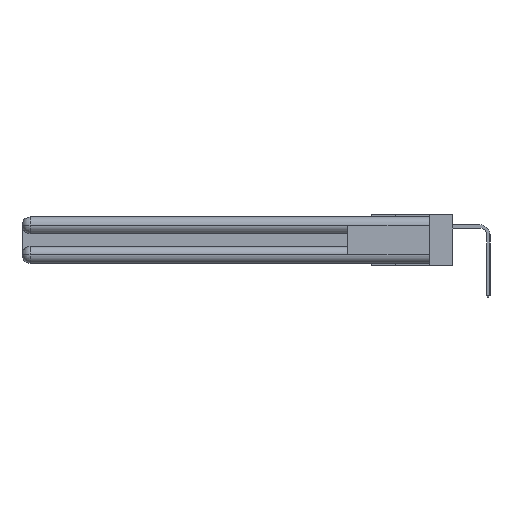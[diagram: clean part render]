
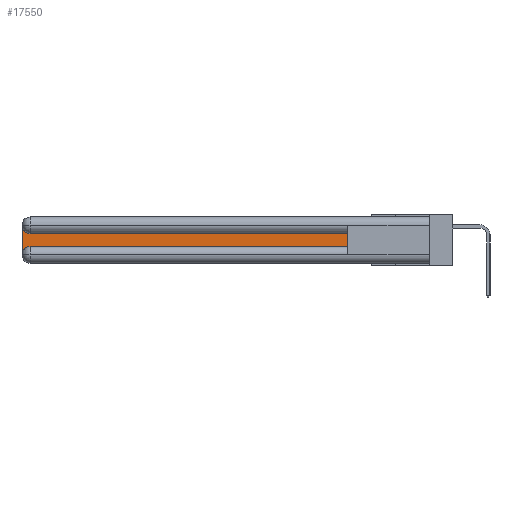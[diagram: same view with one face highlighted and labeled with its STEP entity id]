
A CAD part, left-side view. The second image highlights one B-rep face of the part: STEP entity #17550.
In plain terms, the highlighted planar face has unit normal (-1, 0, 0).
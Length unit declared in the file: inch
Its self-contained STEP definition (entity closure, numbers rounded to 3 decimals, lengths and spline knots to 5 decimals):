
#443 = EDGE_CURVE ( 'NONE', #10282, #14341, #23832, .T. ) ;
#1034 = VERTEX_POINT ( 'NONE', #18353 ) ;
#1280 = CARTESIAN_POINT ( 'NONE',  ( 0.075, 2.94, -0.0625 ) ) ;
#1886 = EDGE_CURVE ( 'NONE', #11792, #10282, #18572, .T. ) ;
#2199 = LINE ( 'NONE', #7753, #11825 ) ;
#2789 = VECTOR ( 'NONE', #24992, 39.37008 ) ;
#3141 = CARTESIAN_POINT ( 'NONE',  ( 0.075, 0.6, -0.2175 ) ) ;
#3787 = CARTESIAN_POINT ( 'NONE',  ( 0.075, 2.94, -0.2775 ) ) ;
#4135 = AXIS2_PLACEMENT_3D ( 'NONE', #23083, #14663, #4190 ) ;
#4190 = DIRECTION ( 'NONE',  ( 0., 0., -1. ) ) ;
#4369 = VECTOR ( 'NONE', #4747, 39.37008 ) ;
#4747 = DIRECTION ( 'NONE',  ( 0., 0., -1. ) ) ;
#5573 = CARTESIAN_POINT ( 'NONE',  ( 0.075, 2.94, -0.2175 ) ) ;
#6013 = DIRECTION ( 'NONE',  ( 0., 0., -1. ) ) ;
#6859 = EDGE_CURVE ( 'NONE', #26523, #1034, #24664, .T. ) ;
#7753 = CARTESIAN_POINT ( 'NONE',  ( 0.075, 0.6, -0.2175 ) ) ;
#9432 = DIRECTION ( 'NONE',  ( 0., 0., 1. ) ) ;
#9988 = CARTESIAN_POINT ( 'NONE',  ( 0.075, 2.94, -0.1225 ) ) ;
#10282 = VERTEX_POINT ( 'NONE', #17084 ) ;
#10383 = FACE_OUTER_BOUND ( 'NONE', #17422, .T. ) ;
#11764 = DIRECTION ( 'NONE',  ( 0., 0., -1. ) ) ;
#11792 = VERTEX_POINT ( 'NONE', #23439 ) ;
#11825 = VECTOR ( 'NONE', #24594, 39.37008 ) ;
#12005 = ORIENTED_EDGE ( 'NONE', *, *, #15302, .T. ) ;
#12708 = EDGE_CURVE ( 'NONE', #13129, #11792, #18549, .T. ) ;
#13129 = VERTEX_POINT ( 'NONE', #9988 ) ;
#14341 = VERTEX_POINT ( 'NONE', #5573 ) ;
#14663 = DIRECTION ( 'NONE',  ( 1., 0., 0. ) ) ;
#15302 = EDGE_CURVE ( 'NONE', #14341, #26523, #2199, .T. ) ;
#15582 = AXIS2_PLACEMENT_3D ( 'NONE', #1280, #16181, #11764 ) ;
#16181 = DIRECTION ( 'NONE',  ( 1., 0., 0. ) ) ;
#17082 = EDGE_CURVE ( 'NONE', #1034, #13129, #25515, .T. ) ;
#17084 = CARTESIAN_POINT ( 'NONE',  ( 0.075, 3., -0.2775 ) ) ;
#17129 = VECTOR ( 'NONE', #9432, 39.37008 ) ;
#17422 = EDGE_LOOP ( 'NONE', ( #19670, #23113, #25956, #22441, #12005, #19313 ) ) ;
#17550 = ADVANCED_FACE ( 'NONE', ( #10383 ), #20731, .F. ) ;
#18353 = CARTESIAN_POINT ( 'NONE',  ( 0.075, 0.6, -0.1225 ) ) ;
#18480 = DIRECTION ( 'NONE',  ( 1., 0., 0. ) ) ;
#18549 = CIRCLE ( 'NONE', #15582, 0.06 ) ;
#18572 = LINE ( 'NONE', #19777, #4369 ) ;
#19313 = ORIENTED_EDGE ( 'NONE', *, *, #6859, .T. ) ;
#19670 = ORIENTED_EDGE ( 'NONE', *, *, #17082, .T. ) ;
#19777 = CARTESIAN_POINT ( 'NONE',  ( 0.075, 3., -0.2175 ) ) ;
#20731 = PLANE ( 'NONE',  #4135 ) ;
#20855 = CARTESIAN_POINT ( 'NONE',  ( 0.075, 0.6, -0.2175 ) ) ;
#22441 = ORIENTED_EDGE ( 'NONE', *, *, #443, .T. ) ;
#23083 = CARTESIAN_POINT ( 'NONE',  ( 0.075, 3., -0.1225 ) ) ;
#23113 = ORIENTED_EDGE ( 'NONE', *, *, #12708, .T. ) ;
#23439 = CARTESIAN_POINT ( 'NONE',  ( 0.075, 3., -0.0625 ) ) ;
#23832 = CIRCLE ( 'NONE', #25921, 0.06 ) ;
#24594 = DIRECTION ( 'NONE',  ( 0., -1., 0. ) ) ;
#24664 = LINE ( 'NONE', #3141, #17129 ) ;
#24992 = DIRECTION ( 'NONE',  ( 0., 1., 0. ) ) ;
#25515 = LINE ( 'NONE', #26993, #2789 ) ;
#25921 = AXIS2_PLACEMENT_3D ( 'NONE', #3787, #18480, #6013 ) ;
#25956 = ORIENTED_EDGE ( 'NONE', *, *, #1886, .T. ) ;
#26523 = VERTEX_POINT ( 'NONE', #20855 ) ;
#26993 = CARTESIAN_POINT ( 'NONE',  ( 0.075, 0.6, -0.1225 ) ) ;
